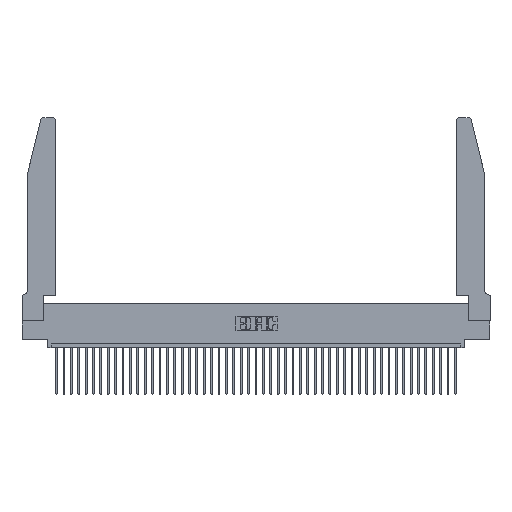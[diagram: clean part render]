
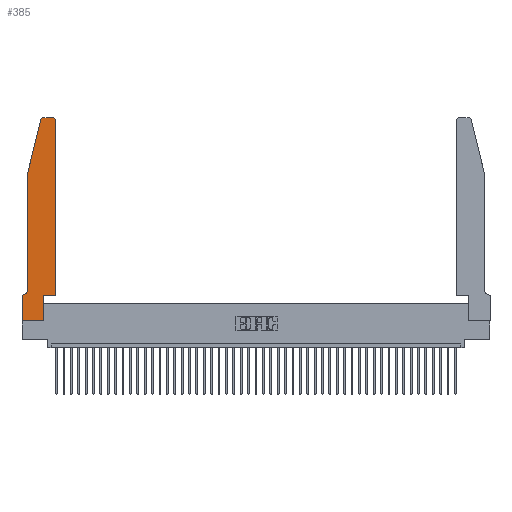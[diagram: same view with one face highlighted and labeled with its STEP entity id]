
A CAD part, top view. The second image highlights one B-rep face of the part: STEP entity #385.
In plain terms, the highlighted planar face has unit normal (0, 0, 1).
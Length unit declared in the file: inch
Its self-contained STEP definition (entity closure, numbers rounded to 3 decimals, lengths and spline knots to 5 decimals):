
#350 = CARTESIAN_POINT ( 'NONE',  ( 0.25487, 2.72718, 0.37 ) ) ;
#385 = ADVANCED_FACE ( 'NONE', ( #27863 ), #22448, .T. ) ;
#524 = ORIENTED_EDGE ( 'NONE', *, *, #43614, .T. ) ;
#1463 = VECTOR ( 'NONE', #36905, 39.37008 ) ;
#1518 = CARTESIAN_POINT ( 'NONE',  ( 0.0055, 0.42, 0.37 ) ) ;
#1717 = EDGE_CURVE ( 'NONE', #4328, #39172, #32074, .T. ) ;
#1758 = CARTESIAN_POINT ( 'NONE',  ( 0.284, 2.72, 0.37 ) ) ;
#1791 = ORIENTED_EDGE ( 'NONE', *, *, #31508, .T. ) ;
#1815 = CARTESIAN_POINT ( 'NONE',  ( 0.2865, 0.35, 0.37 ) ) ;
#1897 = DIRECTION ( 'NONE',  ( 0., 0., 1. ) ) ;
#2201 = CARTESIAN_POINT ( 'NONE',  ( 0., 0.35, 0.37 ) ) ;
#2922 = ORIENTED_EDGE ( 'NONE', *, *, #15120, .T. ) ;
#2969 = AXIS2_PLACEMENT_3D ( 'NONE', #1758, #5208, #44002 ) ;
#3108 = ORIENTED_EDGE ( 'NONE', *, *, #9325, .T. ) ;
#3679 = DIRECTION ( 'NONE',  ( 1., 0., 0. ) ) ;
#3859 = CARTESIAN_POINT ( 'NONE',  ( 0.0055, 0.35, 0.37 ) ) ;
#3938 = LINE ( 'NONE', #23573, #39442 ) ;
#4049 = AXIS2_PLACEMENT_3D ( 'NONE', #8621, #39826, #3679 ) ;
#4328 = VERTEX_POINT ( 'NONE', #11684 ) ;
#4350 = CARTESIAN_POINT ( 'NONE',  ( 0.4205, 2.75, 0.37 ) ) ;
#4490 = EDGE_CURVE ( 'NONE', #39172, #28716, #10789, .T. ) ;
#4958 = DIRECTION ( 'NONE',  ( -1., 0., 0. ) ) ;
#5208 = DIRECTION ( 'NONE',  ( 0., 0., 1. ) ) ;
#5362 = VERTEX_POINT ( 'NONE', #28318 ) ;
#5476 = EDGE_CURVE ( 'NONE', #28716, #43954, #32351, .T. ) ;
#5669 = DIRECTION ( 'NONE',  ( 0., 1., 0. ) ) ;
#5718 = LINE ( 'NONE', #15878, #6787 ) ;
#5883 = ORIENTED_EDGE ( 'NONE', *, *, #17600, .T. ) ;
#6787 = VECTOR ( 'NONE', #5669, 39.37008 ) ;
#6905 = DIRECTION ( 'NONE',  ( -0.239, -0.971, 0. ) ) ;
#6920 = DIRECTION ( 'NONE',  ( 0., -1., 0. ) ) ;
#7305 = ORIENTED_EDGE ( 'NONE', *, *, #1717, .T. ) ;
#7705 = EDGE_CURVE ( 'NONE', #15936, #9752, #22976, .T. ) ;
#7911 = CARTESIAN_POINT ( 'NONE',  ( 0., 0., 0.37 ) ) ;
#7927 = ORIENTED_EDGE ( 'NONE', *, *, #5476, .T. ) ;
#8621 = CARTESIAN_POINT ( 'NONE',  ( 0.4205, 2.72, 0.37 ) ) ;
#9325 = EDGE_CURVE ( 'NONE', #32888, #35606, #3938, .T. ) ;
#9752 = VERTEX_POINT ( 'NONE', #39071 ) ;
#9979 = CARTESIAN_POINT ( 'NONE',  ( 0.4505, 0.35, 0.37 ) ) ;
#10156 = ORIENTED_EDGE ( 'NONE', *, *, #7705, .T. ) ;
#10426 = EDGE_CURVE ( 'NONE', #43954, #36602, #22774, .T. ) ;
#10508 = VERTEX_POINT ( 'NONE', #13403 ) ;
#10789 = LINE ( 'NONE', #44011, #18878 ) ;
#11032 = AXIS2_PLACEMENT_3D ( 'NONE', #1518, #43476, #34306 ) ;
#11684 = CARTESIAN_POINT ( 'NONE',  ( 0.4505, 2.72, 0.37 ) ) ;
#13024 = VECTOR ( 'NONE', #6905, 39.37008 ) ;
#13349 = VECTOR ( 'NONE', #4958, 39.37008 ) ;
#13403 = CARTESIAN_POINT ( 'NONE',  ( 0.0755, 0.42, 0.37 ) ) ;
#13765 = VECTOR ( 'NONE', #28968, 39.37008 ) ;
#15120 = EDGE_CURVE ( 'NONE', #10508, #37868, #36222, .T. ) ;
#15878 = CARTESIAN_POINT ( 'NONE',  ( 0.2865, 0.35, 0.37 ) ) ;
#15936 = VERTEX_POINT ( 'NONE', #25482 ) ;
#17177 = DIRECTION ( 'NONE',  ( 1., 0., 0. ) ) ;
#17257 = VECTOR ( 'NONE', #32068, 39.37008 ) ;
#17600 = EDGE_CURVE ( 'NONE', #37868, #5362, #18213, .T. ) ;
#18213 = LINE ( 'NONE', #35839, #13349 ) ;
#18878 = VECTOR ( 'NONE', #20455, 39.37008 ) ;
#20455 = DIRECTION ( 'NONE',  ( -1., 0., 0. ) ) ;
#22302 = EDGE_CURVE ( 'NONE', #35606, #4328, #23078, .T. ) ;
#22448 = PLANE ( 'NONE',  #32747 ) ;
#22774 = LINE ( 'NONE', #34619, #13024 ) ;
#22976 = LINE ( 'NONE', #42595, #13765 ) ;
#23078 = LINE ( 'NONE', #9979, #1463 ) ;
#23573 = CARTESIAN_POINT ( 'NONE',  ( 0.4505, 0.35, 0.37 ) ) ;
#25162 = CARTESIAN_POINT ( 'NONE',  ( 0.284, 2.75, 0.37 ) ) ;
#25482 = CARTESIAN_POINT ( 'NONE',  ( 0., 0., 0.37 ) ) ;
#25842 = VECTOR ( 'NONE', #6920, 39.37008 ) ;
#27536 = ORIENTED_EDGE ( 'NONE', *, *, #10426, .T. ) ;
#27863 = FACE_OUTER_BOUND ( 'NONE', #42520, .T. ) ;
#28318 = CARTESIAN_POINT ( 'NONE',  ( 0., 0.35, 0.37 ) ) ;
#28716 = VERTEX_POINT ( 'NONE', #25162 ) ;
#28968 = DIRECTION ( 'NONE',  ( 1., 0., 0. ) ) ;
#30476 = CARTESIAN_POINT ( 'NONE',  ( 0.0755, 2., 0.37 ) ) ;
#31403 = ORIENTED_EDGE ( 'NONE', *, *, #22302, .T. ) ;
#31508 = EDGE_CURVE ( 'NONE', #5362, #15936, #38779, .T. ) ;
#32068 = DIRECTION ( 'NONE',  ( 0., -1., 0. ) ) ;
#32074 = CIRCLE ( 'NONE', #4049, 0.03 ) ;
#32351 = CIRCLE ( 'NONE', #2969, 0.03 ) ;
#32747 = AXIS2_PLACEMENT_3D ( 'NONE', #2201, #1897, #43400 ) ;
#32888 = VERTEX_POINT ( 'NONE', #1815 ) ;
#33728 = ORIENTED_EDGE ( 'NONE', *, *, #4490, .T. ) ;
#34306 = DIRECTION ( 'NONE',  ( -1., 0., 0. ) ) ;
#34386 = CARTESIAN_POINT ( 'NONE',  ( 0.4505, 0.35, 0.37 ) ) ;
#34619 = CARTESIAN_POINT ( 'NONE',  ( 0.0755, 2., 0.37 ) ) ;
#35440 = ORIENTED_EDGE ( 'NONE', *, *, #43027, .T. ) ;
#35606 = VERTEX_POINT ( 'NONE', #34386 ) ;
#35839 = CARTESIAN_POINT ( 'NONE',  ( 0.0755, 0.35, 0.37 ) ) ;
#36222 = CIRCLE ( 'NONE', #11032, 0.07 ) ;
#36602 = VERTEX_POINT ( 'NONE', #40455 ) ;
#36905 = DIRECTION ( 'NONE',  ( 0., 1., 0. ) ) ;
#37868 = VERTEX_POINT ( 'NONE', #3859 ) ;
#38779 = LINE ( 'NONE', #7911, #17257 ) ;
#39071 = CARTESIAN_POINT ( 'NONE',  ( 0.2865, 0., 0.37 ) ) ;
#39172 = VERTEX_POINT ( 'NONE', #4350 ) ;
#39442 = VECTOR ( 'NONE', #17177, 39.37008 ) ;
#39826 = DIRECTION ( 'NONE',  ( 0., 0., 1. ) ) ;
#40455 = CARTESIAN_POINT ( 'NONE',  ( 0.0755, 2., 0.37 ) ) ;
#42520 = EDGE_LOOP ( 'NONE', ( #33728, #7927, #27536, #35440, #2922, #5883, #1791, #10156, #524, #3108, #31403, #7305 ) ) ;
#42595 = CARTESIAN_POINT ( 'NONE',  ( 0., 0., 0.37 ) ) ;
#43027 = EDGE_CURVE ( 'NONE', #36602, #10508, #43511, .T. ) ;
#43400 = DIRECTION ( 'NONE',  ( 1., 0., 0. ) ) ;
#43476 = DIRECTION ( 'NONE',  ( 0., 0., -1. ) ) ;
#43511 = LINE ( 'NONE', #30476, #25842 ) ;
#43614 = EDGE_CURVE ( 'NONE', #9752, #32888, #5718, .T. ) ;
#43954 = VERTEX_POINT ( 'NONE', #350 ) ;
#44002 = DIRECTION ( 'NONE',  ( 1., 0., 0. ) ) ;
#44011 = CARTESIAN_POINT ( 'NONE',  ( 0.2605, 2.75, 0.37 ) ) ;
